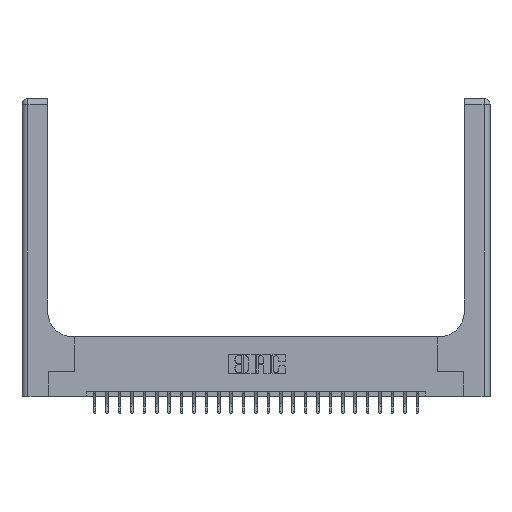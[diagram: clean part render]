
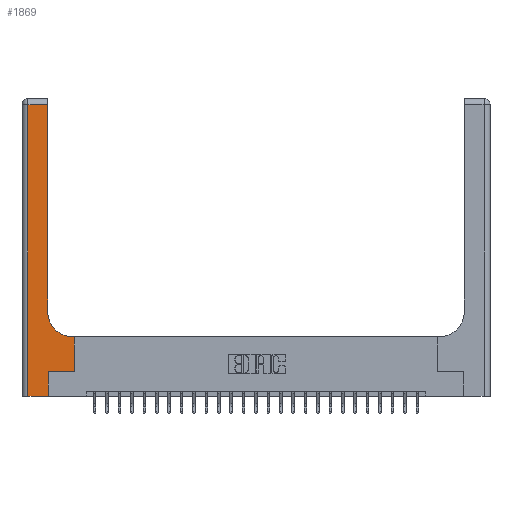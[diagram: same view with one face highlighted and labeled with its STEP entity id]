
A CAD part, top view. The second image highlights one B-rep face of the part: STEP entity #1869.
In plain terms, the highlighted planar face has unit normal (0, 0, 1).
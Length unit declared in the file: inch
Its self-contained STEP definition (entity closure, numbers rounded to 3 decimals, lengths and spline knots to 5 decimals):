
#489 = EDGE_LOOP ( 'NONE', ( #11579, #17207, #14393, #21127, #8752, #18377, #16498, #9569, #16281 ) ) ;
#1038 = CARTESIAN_POINT ( 'NONE',  ( 0.528, 0.25, 0.37 ) ) ;
#1108 = DIRECTION ( 'NONE',  ( 1., 0., 0. ) ) ;
#1162 = VERTEX_POINT ( 'NONE', #5522 ) ;
#1699 = CARTESIAN_POINT ( 'NONE',  ( 0.06, 2.94, 0.37 ) ) ;
#1869 = ADVANCED_FACE ( 'NONE', ( #13084 ), #6418, .F. ) ;
#1975 = VECTOR ( 'NONE', #8968, 39.37008 ) ;
#3053 = CARTESIAN_POINT ( 'NONE',  ( 0., 0., 0.37 ) ) ;
#3243 = DIRECTION ( 'NONE',  ( -1., 0., 0. ) ) ;
#3907 = CARTESIAN_POINT ( 'NONE',  ( 0.265, 0.25, 0.37 ) ) ;
#4628 = CARTESIAN_POINT ( 'NONE',  ( 0.265, 0., 0.37 ) ) ;
#5074 = EDGE_CURVE ( 'NONE', #17572, #1162, #13248, .T. ) ;
#5131 = VERTEX_POINT ( 'NONE', #5218 ) ;
#5218 = CARTESIAN_POINT ( 'NONE',  ( 0.06, 0., 0.37 ) ) ;
#5522 = CARTESIAN_POINT ( 'NONE',  ( 0.528, 0.25, 0.37 ) ) ;
#5531 = LINE ( 'NONE', #1038, #20431 ) ;
#5688 = VECTOR ( 'NONE', #15457, 39.37008 ) ;
#6037 = VERTEX_POINT ( 'NONE', #1699 ) ;
#6418 = PLANE ( 'NONE',  #20784 ) ;
#7004 = LINE ( 'NONE', #14995, #23381 ) ;
#7536 = VERTEX_POINT ( 'NONE', #21118 ) ;
#8325 = LINE ( 'NONE', #3053, #1975 ) ;
#8752 = ORIENTED_EDGE ( 'NONE', *, *, #16535, .T. ) ;
#8874 = VERTEX_POINT ( 'NONE', #15279 ) ;
#8968 = DIRECTION ( 'NONE',  ( 1., 0., 0. ) ) ;
#9120 = DIRECTION ( 'NONE',  ( 0., 0., -1. ) ) ;
#9200 = AXIS2_PLACEMENT_3D ( 'NONE', #18255, #12362, #10595 ) ;
#9542 = LINE ( 'NONE', #11811, #5688 ) ;
#9569 = ORIENTED_EDGE ( 'NONE', *, *, #24143, .T. ) ;
#10247 = VERTEX_POINT ( 'NONE', #20975 ) ;
#10595 = DIRECTION ( 'NONE',  ( 1., 0., 0. ) ) ;
#11579 = ORIENTED_EDGE ( 'NONE', *, *, #13131, .T. ) ;
#11623 = CARTESIAN_POINT ( 'NONE',  ( 0.26, 0.85, 0.37 ) ) ;
#11811 = CARTESIAN_POINT ( 'NONE',  ( 0.26, 3., 0.37 ) ) ;
#11907 = CIRCLE ( 'NONE', #9200, 0.25 ) ;
#12362 = DIRECTION ( 'NONE',  ( 0., 0., -1. ) ) ;
#12430 = CARTESIAN_POINT ( 'NONE',  ( 0., 3., 0.37 ) ) ;
#13084 = FACE_OUTER_BOUND ( 'NONE', #489, .T. ) ;
#13131 = EDGE_CURVE ( 'NONE', #17474, #10247, #9542, .T. ) ;
#13248 = LINE ( 'NONE', #18302, #24826 ) ;
#13272 = VERTEX_POINT ( 'NONE', #4628 ) ;
#14279 = DIRECTION ( 'NONE',  ( -1., 0., 0. ) ) ;
#14393 = ORIENTED_EDGE ( 'NONE', *, *, #18192, .T. ) ;
#14718 = DIRECTION ( 'NONE',  ( 0., 1., 0. ) ) ;
#14995 = CARTESIAN_POINT ( 'NONE',  ( 0.06, 3., 0.37 ) ) ;
#15279 = CARTESIAN_POINT ( 'NONE',  ( 0.51, 0.6, 0.37 ) ) ;
#15431 = LINE ( 'NONE', #18047, #16998 ) ;
#15457 = DIRECTION ( 'NONE',  ( 0., 1., 0. ) ) ;
#15691 = DIRECTION ( 'NONE',  ( -1., 0., 0. ) ) ;
#15787 = EDGE_CURVE ( 'NONE', #8874, #17474, #11907, .T. ) ;
#16252 = CARTESIAN_POINT ( 'NONE',  ( 0.265, 0., 0.37 ) ) ;
#16281 = ORIENTED_EDGE ( 'NONE', *, *, #15787, .T. ) ;
#16498 = ORIENTED_EDGE ( 'NONE', *, *, #21759, .T. ) ;
#16502 = DIRECTION ( 'NONE',  ( 0., 1., 0. ) ) ;
#16535 = EDGE_CURVE ( 'NONE', #13272, #17572, #22275, .T. ) ;
#16998 = VECTOR ( 'NONE', #14279, 39.37008 ) ;
#17091 = VECTOR ( 'NONE', #14718, 39.37008 ) ;
#17207 = ORIENTED_EDGE ( 'NONE', *, *, #17754, .T. ) ;
#17474 = VERTEX_POINT ( 'NONE', #11623 ) ;
#17572 = VERTEX_POINT ( 'NONE', #3907 ) ;
#17754 = EDGE_CURVE ( 'NONE', #10247, #6037, #21892, .T. ) ;
#18047 = CARTESIAN_POINT ( 'NONE',  ( 0.26, 0.6, 0.37 ) ) ;
#18192 = EDGE_CURVE ( 'NONE', #6037, #5131, #7004, .T. ) ;
#18255 = CARTESIAN_POINT ( 'NONE',  ( 0.51, 0.85, 0.37 ) ) ;
#18302 = CARTESIAN_POINT ( 'NONE',  ( 0.265, 0.25, 0.37 ) ) ;
#18377 = ORIENTED_EDGE ( 'NONE', *, *, #5074, .T. ) ;
#19439 = DIRECTION ( 'NONE',  ( 0., -1., 0. ) ) ;
#20431 = VECTOR ( 'NONE', #16502, 39.37008 ) ;
#20448 = EDGE_CURVE ( 'NONE', #5131, #13272, #8325, .T. ) ;
#20701 = VECTOR ( 'NONE', #15691, 39.37008 ) ;
#20784 = AXIS2_PLACEMENT_3D ( 'NONE', #12430, #9120, #3243 ) ;
#20975 = CARTESIAN_POINT ( 'NONE',  ( 0.26, 2.94, 0.37 ) ) ;
#21118 = CARTESIAN_POINT ( 'NONE',  ( 0.528, 0.6, 0.37 ) ) ;
#21127 = ORIENTED_EDGE ( 'NONE', *, *, #20448, .T. ) ;
#21759 = EDGE_CURVE ( 'NONE', #1162, #7536, #5531, .T. ) ;
#21892 = LINE ( 'NONE', #23777, #20701 ) ;
#22275 = LINE ( 'NONE', #16252, #17091 ) ;
#23381 = VECTOR ( 'NONE', #19439, 39.37008 ) ;
#23777 = CARTESIAN_POINT ( 'NONE',  ( 0., 2.94, 0.37 ) ) ;
#24143 = EDGE_CURVE ( 'NONE', #7536, #8874, #15431, .T. ) ;
#24826 = VECTOR ( 'NONE', #1108, 39.37008 ) ;
